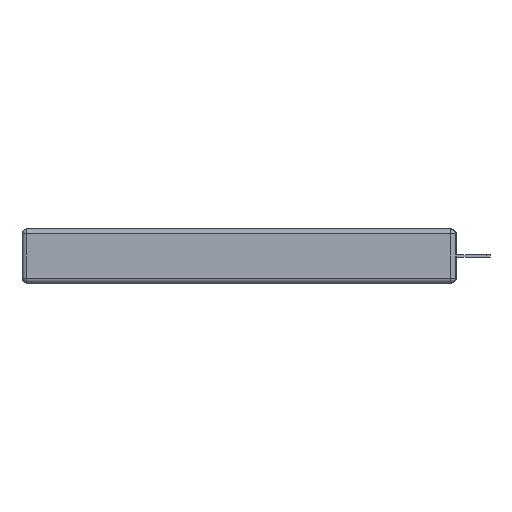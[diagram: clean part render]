
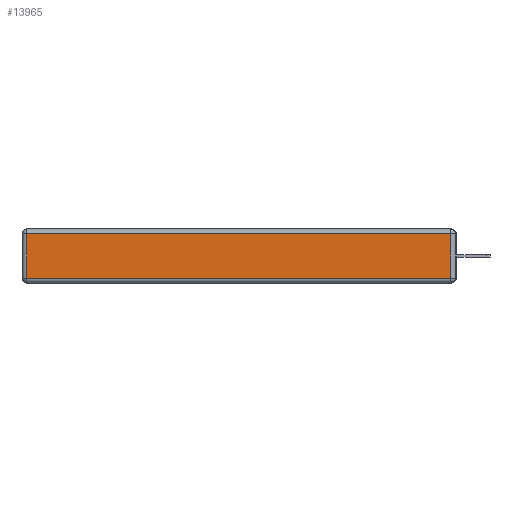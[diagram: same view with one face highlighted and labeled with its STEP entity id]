
A CAD part, left-side view. The second image highlights one B-rep face of the part: STEP entity #13965.
In plain terms, the highlighted planar face has unit normal (-1, 0, 0).
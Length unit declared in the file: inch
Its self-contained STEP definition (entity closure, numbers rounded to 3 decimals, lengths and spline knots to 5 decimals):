
#16 = ORIENTED_EDGE ( 'NONE', *, *, #470, .T. ) ;
#182 = DIRECTION ( 'NONE',  ( 0., 0., 1. ) ) ;
#470 = EDGE_CURVE ( 'NONE', #18263, #12947, #1870, .T. ) ;
#548 = VERTEX_POINT ( 'NONE', #12171 ) ;
#671 = VECTOR ( 'NONE', #10408, 39.37008 ) ;
#1390 = ORIENTED_EDGE ( 'NONE', *, *, #11515, .T. ) ;
#1870 = LINE ( 'NONE', #17986, #671 ) ;
#2280 = CARTESIAN_POINT ( 'NONE',  ( 0., 0., -0.313 ) ) ;
#3001 = LINE ( 'NONE', #6196, #11038 ) ;
#4207 = EDGE_CURVE ( 'NONE', #548, #17172, #3001, .T. ) ;
#6196 = CARTESIAN_POINT ( 'NONE',  ( 0., 0.03, -0.343 ) ) ;
#8570 = VECTOR ( 'NONE', #21792, 39.37008 ) ;
#8873 = CARTESIAN_POINT ( 'NONE',  ( 0., 0.03, -0.03 ) ) ;
#9202 = CARTESIAN_POINT ( 'NONE',  ( 0., 2.75, -0.03 ) ) ;
#10091 = DIRECTION ( 'NONE',  ( 0., 0., 1. ) ) ;
#10408 = DIRECTION ( 'NONE',  ( 0., 0., -1. ) ) ;
#11021 = ORIENTED_EDGE ( 'NONE', *, *, #13331, .T. ) ;
#11038 = VECTOR ( 'NONE', #10091, 39.37008 ) ;
#11086 = DIRECTION ( 'NONE',  ( -1., 0., 0. ) ) ;
#11515 = EDGE_CURVE ( 'NONE', #17172, #18263, #14548, .T. ) ;
#11621 = CARTESIAN_POINT ( 'NONE',  ( 0., 2.72, -0.03 ) ) ;
#12171 = CARTESIAN_POINT ( 'NONE',  ( 0., 0.03, -0.313 ) ) ;
#12947 = VERTEX_POINT ( 'NONE', #20798 ) ;
#13331 = EDGE_CURVE ( 'NONE', #12947, #548, #18513, .T. ) ;
#13965 = ADVANCED_FACE ( 'NONE', ( #22002 ), #16387, .T. ) ;
#14404 = CARTESIAN_POINT ( 'NONE',  ( 0., 0., -0.343 ) ) ;
#14548 = LINE ( 'NONE', #9202, #8570 ) ;
#14725 = AXIS2_PLACEMENT_3D ( 'NONE', #14404, #11086, #182 ) ;
#15573 = ORIENTED_EDGE ( 'NONE', *, *, #4207, .T. ) ;
#16387 = PLANE ( 'NONE',  #14725 ) ;
#17172 = VERTEX_POINT ( 'NONE', #8873 ) ;
#17986 = CARTESIAN_POINT ( 'NONE',  ( 0., 2.72, -0.343 ) ) ;
#18263 = VERTEX_POINT ( 'NONE', #11621 ) ;
#18319 = EDGE_LOOP ( 'NONE', ( #11021, #15573, #1390, #16 ) ) ;
#18513 = LINE ( 'NONE', #2280, #22687 ) ;
#18621 = DIRECTION ( 'NONE',  ( 0., -1., 0. ) ) ;
#20798 = CARTESIAN_POINT ( 'NONE',  ( 0., 2.72, -0.313 ) ) ;
#21792 = DIRECTION ( 'NONE',  ( 0., 1., 0. ) ) ;
#22002 = FACE_OUTER_BOUND ( 'NONE', #18319, .T. ) ;
#22687 = VECTOR ( 'NONE', #18621, 39.37008 ) ;
